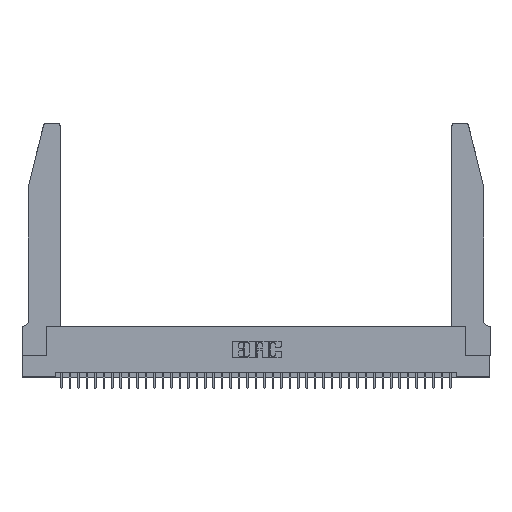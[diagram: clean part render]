
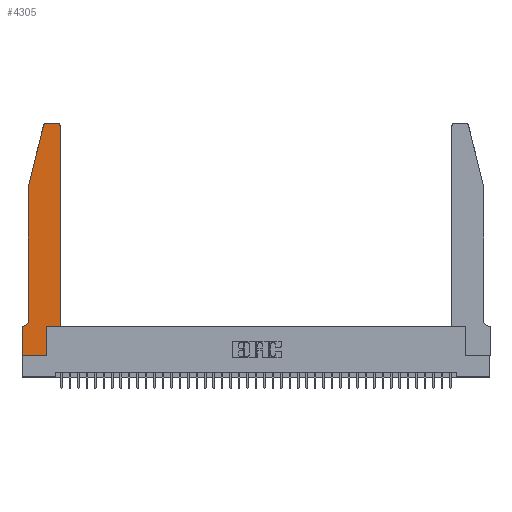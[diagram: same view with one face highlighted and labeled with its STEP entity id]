
A CAD part, top view. The second image highlights one B-rep face of the part: STEP entity #4305.
In plain terms, the highlighted planar face has unit normal (0, 0, 1).
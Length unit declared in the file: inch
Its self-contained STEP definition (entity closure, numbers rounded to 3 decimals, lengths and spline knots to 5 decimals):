
#375 = VERTEX_POINT ( 'NONE', #17696 ) ;
#688 = EDGE_CURVE ( 'NONE', #375, #2649, #19425, .T. ) ;
#708 = VERTEX_POINT ( 'NONE', #38553 ) ;
#1176 = AXIS2_PLACEMENT_3D ( 'NONE', #28646, #37819, #9786 ) ;
#1718 = EDGE_CURVE ( 'NONE', #32509, #18879, #13259, .T. ) ;
#1847 = CARTESIAN_POINT ( 'NONE',  ( 0.4505, 0.35, 0.37 ) ) ;
#2366 = CARTESIAN_POINT ( 'NONE',  ( 0.4205, 2.75, 0.37 ) ) ;
#2649 = VERTEX_POINT ( 'NONE', #4002 ) ;
#3061 = ORIENTED_EDGE ( 'NONE', *, *, #37662, .T. ) ;
#3104 = CARTESIAN_POINT ( 'NONE',  ( 0., 0., 0.37 ) ) ;
#3312 = VERTEX_POINT ( 'NONE', #14331 ) ;
#3562 = CIRCLE ( 'NONE', #40727, 0.07 ) ;
#3571 = AXIS2_PLACEMENT_3D ( 'NONE', #25059, #5554, #36942 ) ;
#4002 = CARTESIAN_POINT ( 'NONE',  ( 0., 0.35, 0.37 ) ) ;
#4305 = ADVANCED_FACE ( 'NONE', ( #31115 ), #5376, .T. ) ;
#4333 = CARTESIAN_POINT ( 'NONE',  ( 0.2605, 2.75, 0.37 ) ) ;
#4496 = CIRCLE ( 'NONE', #1176, 0.03 ) ;
#5376 = PLANE ( 'NONE',  #40197 ) ;
#5449 = VECTOR ( 'NONE', #16092, 39.37008 ) ;
#5554 = DIRECTION ( 'NONE',  ( 0., 0., 1. ) ) ;
#6081 = ORIENTED_EDGE ( 'NONE', *, *, #33658, .T. ) ;
#6541 = DIRECTION ( 'NONE',  ( 1., 0., 0. ) ) ;
#6847 = CARTESIAN_POINT ( 'NONE',  ( 0.4505, 0.35, 0.37 ) ) ;
#7324 = CARTESIAN_POINT ( 'NONE',  ( 0.2865, 0., 0.37 ) ) ;
#7408 = CARTESIAN_POINT ( 'NONE',  ( 0.0755, 0.42, 0.37 ) ) ;
#7672 = DIRECTION ( 'NONE',  ( -1., 0., 0. ) ) ;
#8423 = ORIENTED_EDGE ( 'NONE', *, *, #16387, .T. ) ;
#8706 = VERTEX_POINT ( 'NONE', #14780 ) ;
#9786 = DIRECTION ( 'NONE',  ( 1., 0., 0. ) ) ;
#9806 = ORIENTED_EDGE ( 'NONE', *, *, #33579, .T. ) ;
#9893 = CARTESIAN_POINT ( 'NONE',  ( 0.0755, 0.35, 0.37 ) ) ;
#10778 = CARTESIAN_POINT ( 'NONE',  ( 0.2865, 0.35, 0.37 ) ) ;
#10948 = VECTOR ( 'NONE', #35516, 39.37008 ) ;
#12002 = VERTEX_POINT ( 'NONE', #7324 ) ;
#12021 = LINE ( 'NONE', #1847, #21367 ) ;
#13184 = CARTESIAN_POINT ( 'NONE',  ( 0., 0., 0.37 ) ) ;
#13259 = LINE ( 'NONE', #22398, #30697 ) ;
#13944 = EDGE_LOOP ( 'NONE', ( #14259, #40710, #15950, #33902, #17021, #26250, #8423, #37317, #9806, #6081, #3061, #35270 ) ) ;
#14174 = CARTESIAN_POINT ( 'NONE',  ( 0.284, 2.75, 0.37 ) ) ;
#14259 = ORIENTED_EDGE ( 'NONE', *, *, #33655, .T. ) ;
#14331 = CARTESIAN_POINT ( 'NONE',  ( 0.25487, 2.72718, 0.37 ) ) ;
#14595 = DIRECTION ( 'NONE',  ( 0., -1., 0. ) ) ;
#14780 = CARTESIAN_POINT ( 'NONE',  ( 0.2865, 0.35, 0.37 ) ) ;
#15115 = DIRECTION ( 'NONE',  ( 1., 0., 0. ) ) ;
#15727 = CARTESIAN_POINT ( 'NONE',  ( 0., 0.35, 0.37 ) ) ;
#15950 = ORIENTED_EDGE ( 'NONE', *, *, #26306, .T. ) ;
#16092 = DIRECTION ( 'NONE',  ( -1., 0., 0. ) ) ;
#16228 = VECTOR ( 'NONE', #7672, 39.37008 ) ;
#16387 = EDGE_CURVE ( 'NONE', #2649, #17370, #34158, .T. ) ;
#16985 = LINE ( 'NONE', #6847, #10948 ) ;
#17021 = ORIENTED_EDGE ( 'NONE', *, *, #39344, .T. ) ;
#17370 = VERTEX_POINT ( 'NONE', #3104 ) ;
#17696 = CARTESIAN_POINT ( 'NONE',  ( 0.0055, 0.35, 0.37 ) ) ;
#18024 = DIRECTION ( 'NONE',  ( 0., 0., 1. ) ) ;
#18351 = CARTESIAN_POINT ( 'NONE',  ( 0., 0., 0.37 ) ) ;
#18397 = DIRECTION ( 'NONE',  ( 0., 0., -1. ) ) ;
#18879 = VERTEX_POINT ( 'NONE', #7408 ) ;
#19425 = LINE ( 'NONE', #9893, #5449 ) ;
#20730 = CARTESIAN_POINT ( 'NONE',  ( 0.4505, 2.72, 0.37 ) ) ;
#21308 = EDGE_CURVE ( 'NONE', #38416, #3312, #4496, .T. ) ;
#21367 = VECTOR ( 'NONE', #24287, 39.37008 ) ;
#21727 = CARTESIAN_POINT ( 'NONE',  ( 0.0055, 0.42, 0.37 ) ) ;
#22398 = CARTESIAN_POINT ( 'NONE',  ( 0.0755, 2., 0.37 ) ) ;
#22726 = LINE ( 'NONE', #13184, #26636 ) ;
#24287 = DIRECTION ( 'NONE',  ( 0., 1., 0. ) ) ;
#24760 = VECTOR ( 'NONE', #32173, 39.37008 ) ;
#25019 = LINE ( 'NONE', #30622, #30619 ) ;
#25059 = CARTESIAN_POINT ( 'NONE',  ( 0.4205, 2.72, 0.37 ) ) ;
#25925 = DIRECTION ( 'NONE',  ( 0., -1., 0. ) ) ;
#26250 = ORIENTED_EDGE ( 'NONE', *, *, #688, .T. ) ;
#26269 = VECTOR ( 'NONE', #14595, 39.37008 ) ;
#26306 = EDGE_CURVE ( 'NONE', #3312, #32509, #25019, .T. ) ;
#26524 = EDGE_CURVE ( 'NONE', #17370, #12002, #22726, .T. ) ;
#26636 = VECTOR ( 'NONE', #6541, 39.37008 ) ;
#27427 = CIRCLE ( 'NONE', #3571, 0.03 ) ;
#27711 = CARTESIAN_POINT ( 'NONE',  ( 0.0755, 2., 0.37 ) ) ;
#28646 = CARTESIAN_POINT ( 'NONE',  ( 0.284, 2.72, 0.37 ) ) ;
#29233 = LINE ( 'NONE', #10778, #24760 ) ;
#29953 = VERTEX_POINT ( 'NONE', #20730 ) ;
#30619 = VECTOR ( 'NONE', #33563, 39.37008 ) ;
#30622 = CARTESIAN_POINT ( 'NONE',  ( 0.0755, 2., 0.37 ) ) ;
#30697 = VECTOR ( 'NONE', #25925, 39.37008 ) ;
#31062 = DIRECTION ( 'NONE',  ( -1., 0., 0. ) ) ;
#31115 = FACE_OUTER_BOUND ( 'NONE', #13944, .T. ) ;
#32067 = EDGE_CURVE ( 'NONE', #29953, #36746, #27427, .T. ) ;
#32173 = DIRECTION ( 'NONE',  ( 0., 1., 0. ) ) ;
#32509 = VERTEX_POINT ( 'NONE', #27711 ) ;
#33563 = DIRECTION ( 'NONE',  ( -0.239, -0.971, 0. ) ) ;
#33579 = EDGE_CURVE ( 'NONE', #12002, #8706, #29233, .T. ) ;
#33655 = EDGE_CURVE ( 'NONE', #36746, #38416, #38619, .T. ) ;
#33658 = EDGE_CURVE ( 'NONE', #8706, #708, #16985, .T. ) ;
#33902 = ORIENTED_EDGE ( 'NONE', *, *, #1718, .T. ) ;
#34158 = LINE ( 'NONE', #18351, #26269 ) ;
#35270 = ORIENTED_EDGE ( 'NONE', *, *, #32067, .T. ) ;
#35516 = DIRECTION ( 'NONE',  ( 1., 0., 0. ) ) ;
#36746 = VERTEX_POINT ( 'NONE', #2366 ) ;
#36942 = DIRECTION ( 'NONE',  ( 1., 0., 0. ) ) ;
#37317 = ORIENTED_EDGE ( 'NONE', *, *, #26524, .T. ) ;
#37662 = EDGE_CURVE ( 'NONE', #708, #29953, #12021, .T. ) ;
#37819 = DIRECTION ( 'NONE',  ( 0., 0., 1. ) ) ;
#38416 = VERTEX_POINT ( 'NONE', #14174 ) ;
#38553 = CARTESIAN_POINT ( 'NONE',  ( 0.4505, 0.35, 0.37 ) ) ;
#38619 = LINE ( 'NONE', #4333, #16228 ) ;
#39344 = EDGE_CURVE ( 'NONE', #18879, #375, #3562, .T. ) ;
#40197 = AXIS2_PLACEMENT_3D ( 'NONE', #15727, #18024, #15115 ) ;
#40710 = ORIENTED_EDGE ( 'NONE', *, *, #21308, .T. ) ;
#40727 = AXIS2_PLACEMENT_3D ( 'NONE', #21727, #18397, #31062 ) ;
